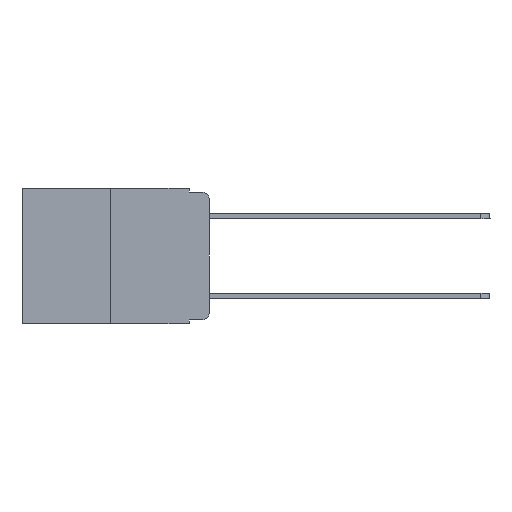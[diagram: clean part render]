
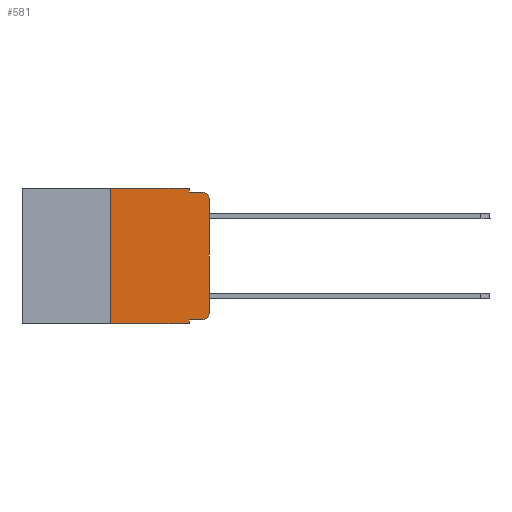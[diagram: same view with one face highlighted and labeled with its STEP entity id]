
A CAD part, left-side view. The second image highlights one B-rep face of the part: STEP entity #581.
In plain terms, the highlighted planar face has unit normal (-1, 0, 0).
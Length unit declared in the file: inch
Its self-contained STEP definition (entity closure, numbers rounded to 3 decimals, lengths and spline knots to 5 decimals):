
#341 = CIRCLE ( 'NONE', #2610, 0.02 ) ;
#394 = CARTESIAN_POINT ( 'NONE',  ( 0., 0.02, -0.333 ) ) ;
#442 = VERTEX_POINT ( 'NONE', #14730 ) ;
#581 = ADVANCED_FACE ( 'NONE', ( #11098 ), #8611, .F. ) ;
#1046 = ORIENTED_EDGE ( 'NONE', *, *, #14912, .T. ) ;
#1119 = VERTEX_POINT ( 'NONE', #4563 ) ;
#1182 = LINE ( 'NONE', #10944, #7126 ) ;
#1300 = EDGE_CURVE ( 'NONE', #8770, #7818, #13532, .T. ) ;
#1366 = ORIENTED_EDGE ( 'NONE', *, *, #5670, .F. ) ;
#1467 = LINE ( 'NONE', #10878, #5712 ) ;
#1702 = ORIENTED_EDGE ( 'NONE', *, *, #14810, .F. ) ;
#2459 = ORIENTED_EDGE ( 'NONE', *, *, #14330, .F. ) ;
#2549 = LINE ( 'NONE', #7913, #4577 ) ;
#2579 = ORIENTED_EDGE ( 'NONE', *, *, #13328, .T. ) ;
#2605 = EDGE_LOOP ( 'NONE', ( #11757, #9123, #1366, #2459, #16597, #1702, #8467, #8326, #1046, #2579 ) ) ;
#2610 = AXIS2_PLACEMENT_3D ( 'NONE', #3872, #7577, #11706 ) ;
#2622 = DIRECTION ( 'NONE',  ( 0., -1., 0. ) ) ;
#2656 = LINE ( 'NONE', #7758, #9189 ) ;
#3582 = CARTESIAN_POINT ( 'NONE',  ( 0., 0.25, 0. ) ) ;
#3872 = CARTESIAN_POINT ( 'NONE',  ( 0., 0.02, -0.03 ) ) ;
#4563 = CARTESIAN_POINT ( 'NONE',  ( 0., 0.051, -0.01 ) ) ;
#4577 = VECTOR ( 'NONE', #13294, 39.37008 ) ;
#5126 = DIRECTION ( 'NONE',  ( 0., -1., 0. ) ) ;
#5530 = LINE ( 'NONE', #8243, #9358 ) ;
#5631 = DIRECTION ( 'NONE',  ( 0., 0., -1. ) ) ;
#5670 = EDGE_CURVE ( 'NONE', #1119, #11274, #2656, .T. ) ;
#5712 = VECTOR ( 'NONE', #14862, 39.37008 ) ;
#5875 = DIRECTION ( 'NONE',  ( -1., 0., 0. ) ) ;
#6087 = CARTESIAN_POINT ( 'NONE',  ( 0., 0., -0.313 ) ) ;
#6096 = VERTEX_POINT ( 'NONE', #7904 ) ;
#6556 = AXIS2_PLACEMENT_3D ( 'NONE', #11158, #5875, #9828 ) ;
#7126 = VECTOR ( 'NONE', #16321, 39.37008 ) ;
#7139 = DIRECTION ( 'NONE',  ( 1., 0., 0. ) ) ;
#7404 = CIRCLE ( 'NONE', #6556, 0.02 ) ;
#7577 = DIRECTION ( 'NONE',  ( -1., 0., 0. ) ) ;
#7627 = VERTEX_POINT ( 'NONE', #10811 ) ;
#7758 = CARTESIAN_POINT ( 'NONE',  ( 0., 0.051, -0.01 ) ) ;
#7818 = VERTEX_POINT ( 'NONE', #10079 ) ;
#7904 = CARTESIAN_POINT ( 'NONE',  ( 0., 0.051, 0. ) ) ;
#7913 = CARTESIAN_POINT ( 'NONE',  ( 0., 0.051, 0. ) ) ;
#8124 = LINE ( 'NONE', #9181, #13731 ) ;
#8243 = CARTESIAN_POINT ( 'NONE',  ( 0., 0.051, -0.333 ) ) ;
#8326 = ORIENTED_EDGE ( 'NONE', *, *, #14467, .F. ) ;
#8422 = EDGE_CURVE ( 'NONE', #11085, #6096, #8124, .T. ) ;
#8467 = ORIENTED_EDGE ( 'NONE', *, *, #15346, .T. ) ;
#8611 = PLANE ( 'NONE',  #14608 ) ;
#8770 = VERTEX_POINT ( 'NONE', #6087 ) ;
#9123 = ORIENTED_EDGE ( 'NONE', *, *, #14251, .T. ) ;
#9181 = CARTESIAN_POINT ( 'NONE',  ( 0., 0.473, 0. ) ) ;
#9189 = VECTOR ( 'NONE', #5126, 39.37008 ) ;
#9210 = DIRECTION ( 'NONE',  ( 0., 0., 1. ) ) ;
#9358 = VECTOR ( 'NONE', #2622, 39.37008 ) ;
#9756 = VECTOR ( 'NONE', #9210, 39.37008 ) ;
#9828 = DIRECTION ( 'NONE',  ( 0., 0., -1. ) ) ;
#10079 = CARTESIAN_POINT ( 'NONE',  ( 0., 0., -0.03 ) ) ;
#10246 = CARTESIAN_POINT ( 'NONE',  ( 0., 0.25, -0.343 ) ) ;
#10755 = VECTOR ( 'NONE', #5631, 39.37008 ) ;
#10811 = CARTESIAN_POINT ( 'NONE',  ( 0., 0.051, -0.333 ) ) ;
#10878 = CARTESIAN_POINT ( 'NONE',  ( 0., 0.25, 0. ) ) ;
#10944 = CARTESIAN_POINT ( 'NONE',  ( 0., 0.473, -0.343 ) ) ;
#11085 = VERTEX_POINT ( 'NONE', #3582 ) ;
#11098 = FACE_OUTER_BOUND ( 'NONE', #2605, .T. ) ;
#11158 = CARTESIAN_POINT ( 'NONE',  ( 0., 0.02, -0.313 ) ) ;
#11274 = VERTEX_POINT ( 'NONE', #16589 ) ;
#11351 = DIRECTION ( 'NONE',  ( 0., 0., -1. ) ) ;
#11706 = DIRECTION ( 'NONE',  ( 0., 0., -1. ) ) ;
#11757 = ORIENTED_EDGE ( 'NONE', *, *, #1300, .T. ) ;
#12138 = LINE ( 'NONE', #12309, #10755 ) ;
#12309 = CARTESIAN_POINT ( 'NONE',  ( 0., 0.051, 0. ) ) ;
#12586 = CARTESIAN_POINT ( 'NONE',  ( 0., 0.473, 0. ) ) ;
#13294 = DIRECTION ( 'NONE',  ( 0., 0., -1. ) ) ;
#13328 = EDGE_CURVE ( 'NONE', #14976, #8770, #7404, .T. ) ;
#13532 = LINE ( 'NONE', #14685, #9756 ) ;
#13731 = VECTOR ( 'NONE', #17380, 39.37008 ) ;
#14251 = EDGE_CURVE ( 'NONE', #7818, #11274, #341, .T. ) ;
#14330 = EDGE_CURVE ( 'NONE', #6096, #1119, #2549, .T. ) ;
#14467 = EDGE_CURVE ( 'NONE', #7627, #442, #12138, .T. ) ;
#14608 = AXIS2_PLACEMENT_3D ( 'NONE', #12586, #7139, #11351 ) ;
#14685 = CARTESIAN_POINT ( 'NONE',  ( 0., 0., 0. ) ) ;
#14730 = CARTESIAN_POINT ( 'NONE',  ( 0., 0.051, -0.343 ) ) ;
#14810 = EDGE_CURVE ( 'NONE', #16497, #11085, #1467, .T. ) ;
#14862 = DIRECTION ( 'NONE',  ( 0., 0., 1. ) ) ;
#14912 = EDGE_CURVE ( 'NONE', #7627, #14976, #5530, .T. ) ;
#14976 = VERTEX_POINT ( 'NONE', #394 ) ;
#15346 = EDGE_CURVE ( 'NONE', #16497, #442, #1182, .T. ) ;
#16321 = DIRECTION ( 'NONE',  ( 0., -1., 0. ) ) ;
#16497 = VERTEX_POINT ( 'NONE', #10246 ) ;
#16589 = CARTESIAN_POINT ( 'NONE',  ( 0., 0.02, -0.01 ) ) ;
#16597 = ORIENTED_EDGE ( 'NONE', *, *, #8422, .F. ) ;
#17380 = DIRECTION ( 'NONE',  ( 0., -1., 0. ) ) ;
